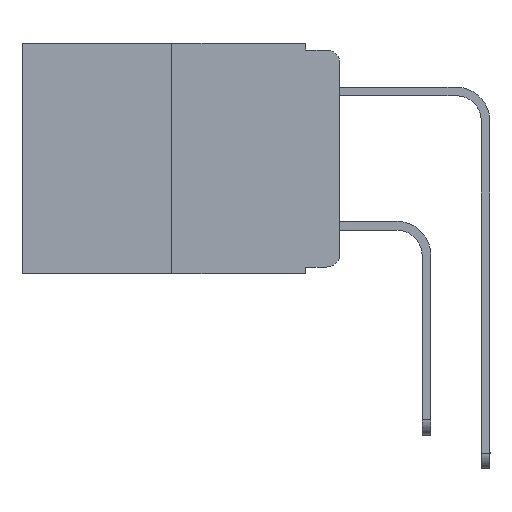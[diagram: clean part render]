
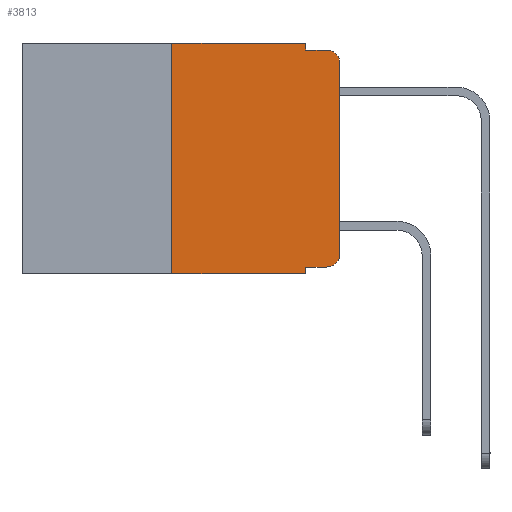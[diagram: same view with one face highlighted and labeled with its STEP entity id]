
A CAD part, left-side view. The second image highlights one B-rep face of the part: STEP entity #3813.
In plain terms, the highlighted planar face has unit normal (-1, 0, 0).
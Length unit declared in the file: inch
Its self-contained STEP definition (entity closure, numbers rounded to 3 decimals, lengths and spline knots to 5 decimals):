
#406 = ORIENTED_EDGE ( 'NONE', *, *, #13998, .F. ) ;
#756 = ORIENTED_EDGE ( 'NONE', *, *, #1143, .F. ) ;
#1049 = VECTOR ( 'NONE', #10922, 39.37008 ) ;
#1096 = LINE ( 'NONE', #13377, #3226 ) ;
#1143 = EDGE_CURVE ( 'NONE', #13839, #12708, #3004, .T. ) ;
#1297 = DIRECTION ( 'NONE',  ( 0., 0., -1. ) ) ;
#1301 = ORIENTED_EDGE ( 'NONE', *, *, #14521, .F. ) ;
#1444 = VECTOR ( 'NONE', #3709, 39.37008 ) ;
#1914 = DIRECTION ( 'NONE',  ( -1., 0., 0. ) ) ;
#2142 = DIRECTION ( 'NONE',  ( 0., 0., -1. ) ) ;
#2603 = CARTESIAN_POINT ( 'NONE',  ( 0., 0.051, -0.01 ) ) ;
#2967 = DIRECTION ( 'NONE',  ( 0., -1., 0. ) ) ;
#2978 = CARTESIAN_POINT ( 'NONE',  ( 0., 0., -0.03 ) ) ;
#3004 = LINE ( 'NONE', #14671, #5711 ) ;
#3226 = VECTOR ( 'NONE', #2142, 39.37008 ) ;
#3557 = EDGE_CURVE ( 'NONE', #12490, #9439, #9219, .T. ) ;
#3622 = VECTOR ( 'NONE', #11251, 39.37008 ) ;
#3709 = DIRECTION ( 'NONE',  ( 0., -1., 0. ) ) ;
#3813 = ADVANCED_FACE ( 'NONE', ( #10504 ), #13819, .F. ) ;
#4167 = VECTOR ( 'NONE', #2967, 39.37008 ) ;
#4205 = DIRECTION ( 'NONE',  ( 0., -1., 0. ) ) ;
#4400 = EDGE_LOOP ( 'NONE', ( #9900, #5998, #9724, #1301, #9104, #756, #12115, #406, #7491, #10332 ) ) ;
#4693 = AXIS2_PLACEMENT_3D ( 'NONE', #5244, #7727, #8833 ) ;
#4877 = VERTEX_POINT ( 'NONE', #2978 ) ;
#5196 = CARTESIAN_POINT ( 'NONE',  ( 0., 0.25, -0.343 ) ) ;
#5239 = LINE ( 'NONE', #14312, #1049 ) ;
#5244 = CARTESIAN_POINT ( 'NONE',  ( 0., 0.02, -0.313 ) ) ;
#5316 = CARTESIAN_POINT ( 'NONE',  ( 0., 0.473, -0.343 ) ) ;
#5625 = LINE ( 'NONE', #12613, #8007 ) ;
#5711 = VECTOR ( 'NONE', #8664, 39.37008 ) ;
#5795 = CARTESIAN_POINT ( 'NONE',  ( 0., 0., 0. ) ) ;
#5998 = ORIENTED_EDGE ( 'NONE', *, *, #14012, .T. ) ;
#6350 = EDGE_CURVE ( 'NONE', #8563, #13380, #8273, .T. ) ;
#6389 = LINE ( 'NONE', #5795, #3622 ) ;
#6782 = CARTESIAN_POINT ( 'NONE',  ( 0., 0., -0.313 ) ) ;
#6975 = EDGE_CURVE ( 'NONE', #13839, #9971, #7569, .T. ) ;
#7081 = CARTESIAN_POINT ( 'NONE',  ( 0., 0.473, 0. ) ) ;
#7328 = CARTESIAN_POINT ( 'NONE',  ( 0., 0.051, -0.01 ) ) ;
#7408 = CARTESIAN_POINT ( 'NONE',  ( 0., 0.02, -0.01 ) ) ;
#7491 = ORIENTED_EDGE ( 'NONE', *, *, #11326, .T. ) ;
#7569 = LINE ( 'NONE', #5316, #9085 ) ;
#7727 = DIRECTION ( 'NONE',  ( -1., 0., 0. ) ) ;
#7750 = CARTESIAN_POINT ( 'NONE',  ( 0., 0.02, -0.03 ) ) ;
#8007 = VECTOR ( 'NONE', #1297, 39.37008 ) ;
#8273 = LINE ( 'NONE', #2603, #1444 ) ;
#8563 = VERTEX_POINT ( 'NONE', #7328 ) ;
#8664 = DIRECTION ( 'NONE',  ( 0., 0., 1. ) ) ;
#8833 = DIRECTION ( 'NONE',  ( 0., 0., -1. ) ) ;
#8967 = VERTEX_POINT ( 'NONE', #9180 ) ;
#9085 = VECTOR ( 'NONE', #4205, 39.37008 ) ;
#9104 = ORIENTED_EDGE ( 'NONE', *, *, #12545, .F. ) ;
#9180 = CARTESIAN_POINT ( 'NONE',  ( 0., 0.051, -0.333 ) ) ;
#9219 = CIRCLE ( 'NONE', #4693, 0.02 ) ;
#9342 = EDGE_CURVE ( 'NONE', #9439, #4877, #6389, .T. ) ;
#9439 = VERTEX_POINT ( 'NONE', #6782 ) ;
#9724 = ORIENTED_EDGE ( 'NONE', *, *, #6350, .F. ) ;
#9814 = CARTESIAN_POINT ( 'NONE',  ( 0., 0.25, 0. ) ) ;
#9900 = ORIENTED_EDGE ( 'NONE', *, *, #9342, .T. ) ;
#9971 = VERTEX_POINT ( 'NONE', #14592 ) ;
#10332 = ORIENTED_EDGE ( 'NONE', *, *, #3557, .T. ) ;
#10504 = FACE_OUTER_BOUND ( 'NONE', #4400, .T. ) ;
#10646 = DIRECTION ( 'NONE',  ( 1., 0., 0. ) ) ;
#10720 = CARTESIAN_POINT ( 'NONE',  ( 0., 0.473, 0. ) ) ;
#10922 = DIRECTION ( 'NONE',  ( 0., -1., 0. ) ) ;
#11003 = CARTESIAN_POINT ( 'NONE',  ( 0., 0.051, 0. ) ) ;
#11251 = DIRECTION ( 'NONE',  ( 0., 0., 1. ) ) ;
#11324 = CIRCLE ( 'NONE', #11567, 0.02 ) ;
#11326 = EDGE_CURVE ( 'NONE', #8967, #12490, #5239, .T. ) ;
#11445 = AXIS2_PLACEMENT_3D ( 'NONE', #7081, #10646, #11678 ) ;
#11567 = AXIS2_PLACEMENT_3D ( 'NONE', #7750, #1914, #12114 ) ;
#11678 = DIRECTION ( 'NONE',  ( 0., 0., -1. ) ) ;
#12114 = DIRECTION ( 'NONE',  ( 0., 0., -1. ) ) ;
#12115 = ORIENTED_EDGE ( 'NONE', *, *, #6975, .T. ) ;
#12490 = VERTEX_POINT ( 'NONE', #12926 ) ;
#12545 = EDGE_CURVE ( 'NONE', #12708, #14437, #13145, .T. ) ;
#12613 = CARTESIAN_POINT ( 'NONE',  ( 0., 0.051, 0. ) ) ;
#12708 = VERTEX_POINT ( 'NONE', #9814 ) ;
#12926 = CARTESIAN_POINT ( 'NONE',  ( 0., 0.02, -0.333 ) ) ;
#13145 = LINE ( 'NONE', #10720, #4167 ) ;
#13377 = CARTESIAN_POINT ( 'NONE',  ( 0., 0.051, 0. ) ) ;
#13380 = VERTEX_POINT ( 'NONE', #7408 ) ;
#13819 = PLANE ( 'NONE',  #11445 ) ;
#13839 = VERTEX_POINT ( 'NONE', #5196 ) ;
#13998 = EDGE_CURVE ( 'NONE', #8967, #9971, #1096, .T. ) ;
#14012 = EDGE_CURVE ( 'NONE', #4877, #13380, #11324, .T. ) ;
#14312 = CARTESIAN_POINT ( 'NONE',  ( 0., 0.051, -0.333 ) ) ;
#14437 = VERTEX_POINT ( 'NONE', #11003 ) ;
#14521 = EDGE_CURVE ( 'NONE', #14437, #8563, #5625, .T. ) ;
#14592 = CARTESIAN_POINT ( 'NONE',  ( 0., 0.051, -0.343 ) ) ;
#14671 = CARTESIAN_POINT ( 'NONE',  ( 0., 0.25, 0. ) ) ;
